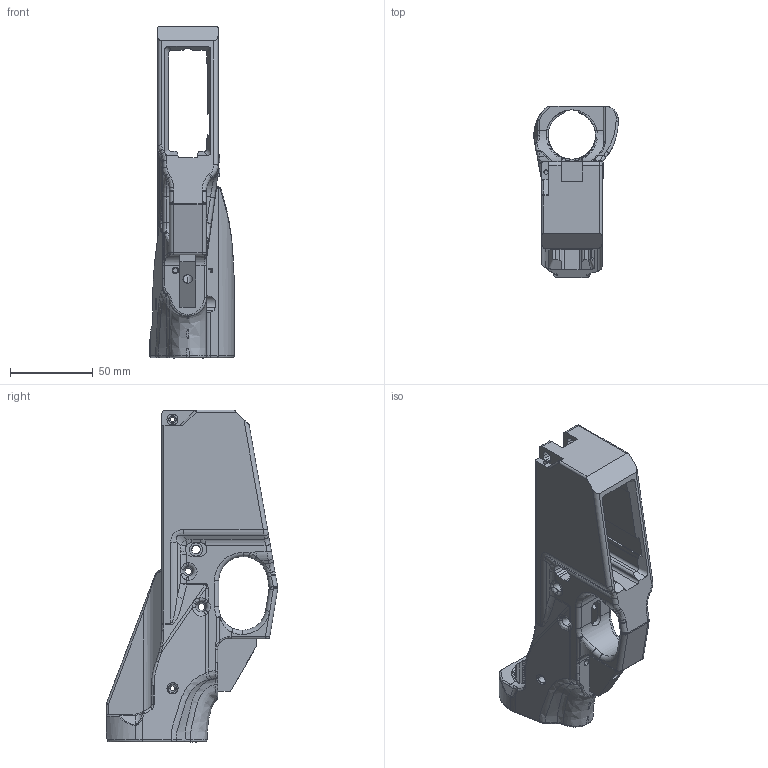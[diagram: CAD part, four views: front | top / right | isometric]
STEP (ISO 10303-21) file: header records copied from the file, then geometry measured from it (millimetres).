
FILE_DESCRIPTION (( 'STEP AP203' ), '1' );
FILE_NAME ('Basic Hoffman Tactical AR-15 Lower.STEP', '2021-03-02T23:45:48', ( 'Frank' ), ( 'Microsoft' ), 'SwSTEP 2.0', 'SolidWorks 2011', '' );
FILE_SCHEMA (( 'CONFIG_CONTROL_DESIGN' ));
Products named in the file (1): Basic Hoffman Tactical AR-15 Lower
Bounding box: 50.8 x 103.34 x 200.03 mm (x, y, z)
Volume: 197703.3 mm3; surface area: 65265.1 mm2
Topology: 1 solids, 1 shells, 711 faces, 1901 edges, 1180 vertices
Faces by surface type: cylinder 263, bspline 186, plane 184, torus 44, cone 22, sphere 12
Entity records: 51279 total; most frequent: CARTESIAN_POINT 35398, ORIENTED_EDGE 3780, DIRECTION 2792, EDGE_CURVE 1890, VERTEX_POINT 1178, AXIS2_PLACEMENT_3D 1033, EDGE_LOOP 748, LINE 726
